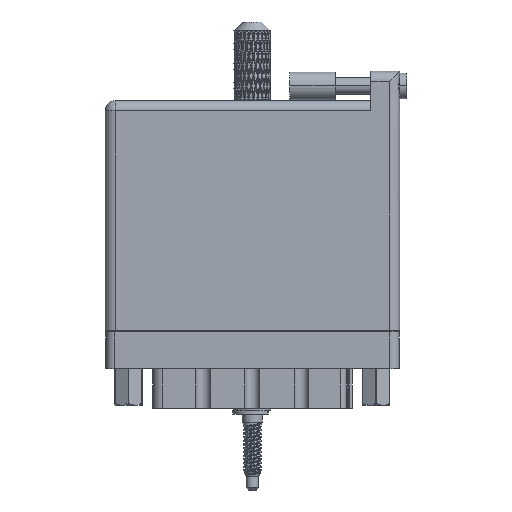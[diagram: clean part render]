
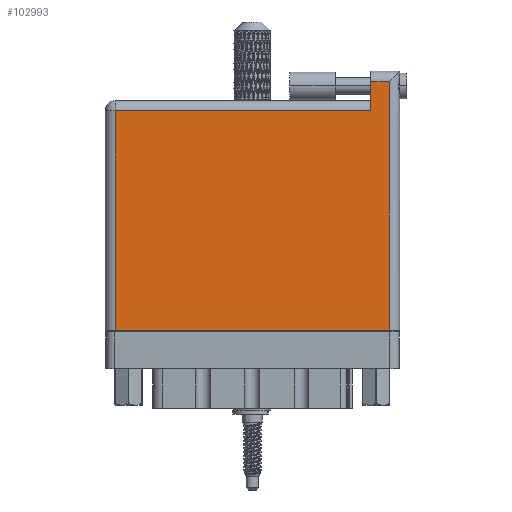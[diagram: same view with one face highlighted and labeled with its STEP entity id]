
A CAD part, front view. The second image highlights one B-rep face of the part: STEP entity #102993.
In plain terms, the highlighted face is planar.
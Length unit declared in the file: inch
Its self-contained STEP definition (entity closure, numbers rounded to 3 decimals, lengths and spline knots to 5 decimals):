
#8635 = EDGE_LOOP ( 'NONE', ( #81717, #12371, #63786, #92178, #23441, #108297 ) ) ;
#11375 = CARTESIAN_POINT ( 'NONE',  ( 0., 1.696, 0. ) ) ;
#12371 = ORIENTED_EDGE ( 'NONE', *, *, #52706, .T. ) ;
#13540 = DIRECTION ( 'NONE',  ( 0., 1., 0. ) ) ;
#13681 = DIRECTION ( 'NONE',  ( -1., 0., 0. ) ) ;
#15772 = CARTESIAN_POINT ( 'NONE',  ( 1.938, 1.696, 0. ) ) ;
#17865 = EDGE_CURVE ( 'NONE', #82973, #56782, #26177, .T. ) ;
#21056 = CARTESIAN_POINT ( 'NONE',  ( 1.811, 1.696, 0. ) ) ;
#22388 = CARTESIAN_POINT ( 'NONE',  ( 1.811, 1.766, 0. ) ) ;
#23441 = ORIENTED_EDGE ( 'NONE', *, *, #103400, .T. ) ;
#23500 = VERTEX_POINT ( 'NONE', #102107 ) ;
#26177 = LINE ( 'NONE', #79961, #48085 ) ;
#27379 = CARTESIAN_POINT ( 'NONE',  ( 1.938, 0., 0. ) ) ;
#33087 = DIRECTION ( 'NONE',  ( 0., -1., 0. ) ) ;
#35092 = VERTEX_POINT ( 'NONE', #15772 ) ;
#35674 = FACE_OUTER_BOUND ( 'NONE', #8635, .T. ) ;
#37264 = DIRECTION ( 'NONE',  ( 1., 0., 0. ) ) ;
#40360 = CARTESIAN_POINT ( 'NONE',  ( 0.07, 0., 0. ) ) ;
#41436 = EDGE_CURVE ( 'NONE', #51592, #82973, #51236, .T. ) ;
#46752 = PLANE ( 'NONE',  #47063 ) ;
#47002 = LINE ( 'NONE', #22388, #100040 ) ;
#47021 = DIRECTION ( 'NONE',  ( -1., 0., 0. ) ) ;
#47063 = AXIS2_PLACEMENT_3D ( 'NONE', #63736, #98803, #90042 ) ;
#48085 = VECTOR ( 'NONE', #37264, 39.37008 ) ;
#51236 = LINE ( 'NONE', #85733, #73704 ) ;
#51592 = VERTEX_POINT ( 'NONE', #72798 ) ;
#52706 = EDGE_CURVE ( 'NONE', #56782, #35092, #111192, .T. ) ;
#54644 = LINE ( 'NONE', #11375, #81875 ) ;
#56782 = VERTEX_POINT ( 'NONE', #27379 ) ;
#57496 = DIRECTION ( 'NONE',  ( 0., -1., 0. ) ) ;
#61459 = EDGE_CURVE ( 'NONE', #35092, #81946, #54644, .T. ) ;
#63736 = CARTESIAN_POINT ( 'NONE',  ( 0., 1.566, 0. ) ) ;
#63786 = ORIENTED_EDGE ( 'NONE', *, *, #61459, .T. ) ;
#72798 = CARTESIAN_POINT ( 'NONE',  ( 0.07, 1.496, 0. ) ) ;
#73704 = VECTOR ( 'NONE', #33087, 39.37008 ) ;
#74966 = CARTESIAN_POINT ( 'NONE',  ( 1.938, 1.766, 0. ) ) ;
#76374 = EDGE_CURVE ( 'NONE', #81946, #23500, #47002, .T. ) ;
#79961 = CARTESIAN_POINT ( 'NONE',  ( 0., 0., 0. ) ) ;
#81717 = ORIENTED_EDGE ( 'NONE', *, *, #17865, .T. ) ;
#81875 = VECTOR ( 'NONE', #47021, 39.37008 ) ;
#81946 = VERTEX_POINT ( 'NONE', #21056 ) ;
#82973 = VERTEX_POINT ( 'NONE', #40360 ) ;
#85733 = CARTESIAN_POINT ( 'NONE',  ( 0.07, 0., 0. ) ) ;
#86743 = CARTESIAN_POINT ( 'NONE',  ( 0., 1.496, 0. ) ) ;
#90042 = DIRECTION ( 'NONE',  ( -1., 0., 0. ) ) ;
#92178 = ORIENTED_EDGE ( 'NONE', *, *, #76374, .T. ) ;
#98803 = DIRECTION ( 'NONE',  ( 0., 0., -1. ) ) ;
#100040 = VECTOR ( 'NONE', #57496, 39.37008 ) ;
#101629 = VECTOR ( 'NONE', #13540, 39.37008 ) ;
#102107 = CARTESIAN_POINT ( 'NONE',  ( 1.811, 1.496, 0. ) ) ;
#102993 = ADVANCED_FACE ( 'NONE', ( #35674 ), #46752, .F. ) ;
#103400 = EDGE_CURVE ( 'NONE', #23500, #51592, #111912, .T. ) ;
#108297 = ORIENTED_EDGE ( 'NONE', *, *, #41436, .T. ) ;
#108736 = VECTOR ( 'NONE', #13681, 39.37008 ) ;
#111192 = LINE ( 'NONE', #74966, #101629 ) ;
#111912 = LINE ( 'NONE', #86743, #108736 ) ;
